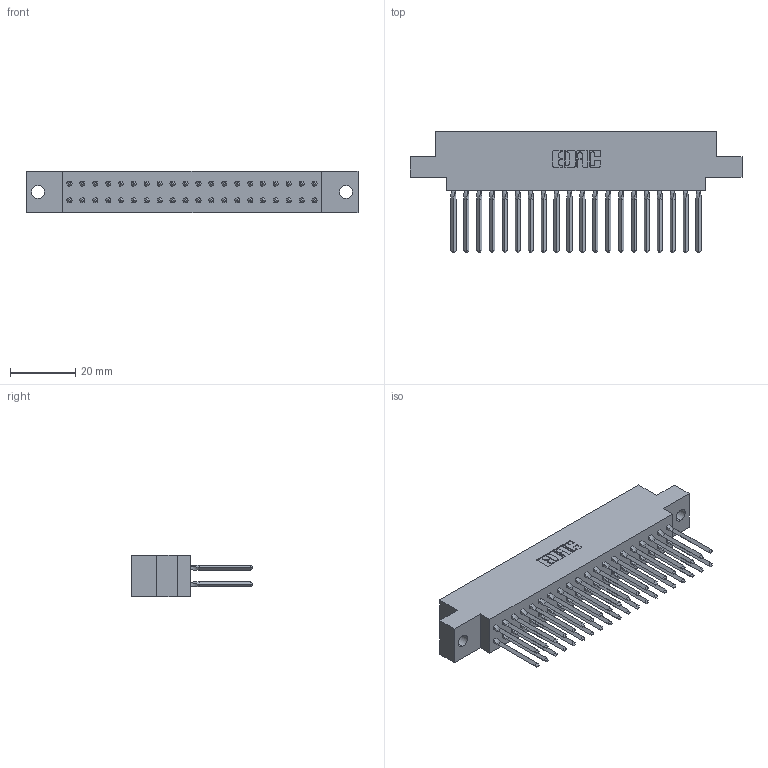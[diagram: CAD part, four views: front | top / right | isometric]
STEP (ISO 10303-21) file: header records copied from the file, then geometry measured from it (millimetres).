
FILE_DESCRIPTION (( 'STEP AP203' ), '1' );
FILE_NAME ('317-040-540-804.STEP', '2020-02-28T00:28:13', ( '' ), ( '' ), 'SwSTEP 2.0', 'SolidWorks 2016', '' );
FILE_SCHEMA (( 'CONFIG_CONTROL_DESIGN' ));
Length unit declared in the file: inch
Products named in the file (3): 317-040-540-804; 317 Part_.156 Dia - TH; 317-290-001_540
Assembly tree (41 placements, depth 2):
  317-040-540-804
    317 Part_.156 Dia - TH
    317-290-001_540  x40
Bounding box: 101.96 x 37.34 x 12.7 mm (x, y, z)
Volume: 16279.6 mm3; surface area: 23265.5 mm2
Topology: 41 solids, 41 shells, 3662 faces, 10155 edges, 6542 vertices
Faces by surface type: plane 2978, cylinder 524, bspline 160
Entity records: 31982 total; most frequent: CARTESIAN_POINT 5991, ORIENTED_EDGE 5490, DIRECTION 4583, EDGE_CURVE 2745, VECTOR 2489, LINE 2489, VERTEX_POINT 1823, AXIS2_PLACEMENT_3D 1047
